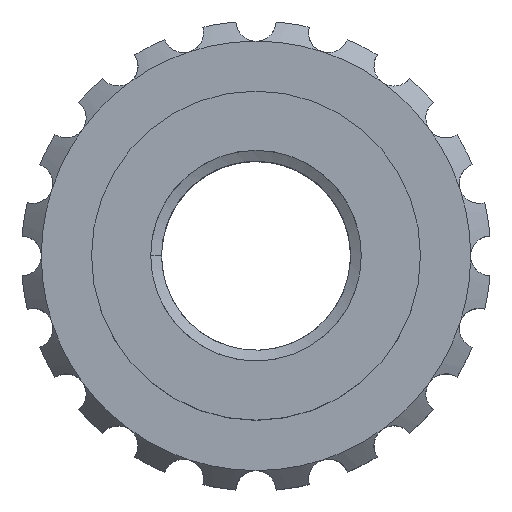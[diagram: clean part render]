
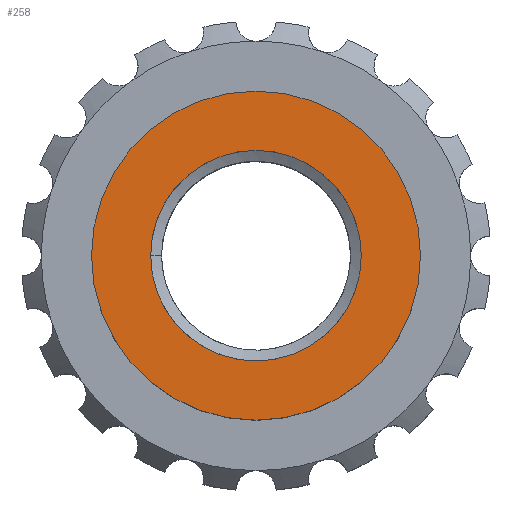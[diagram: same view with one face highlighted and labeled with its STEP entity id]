
A CAD part, top view. The second image highlights one B-rep face of the part: STEP entity #258.
In plain terms, the highlighted planar face has unit normal (0, 0, 1).
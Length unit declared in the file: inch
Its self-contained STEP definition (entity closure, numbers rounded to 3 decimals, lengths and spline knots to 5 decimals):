
#20 = CARTESIAN_POINT ( 'NONE',  ( -1.7725, 0.56133, 0.35 ) ) ;
#68 = CIRCLE ( 'NONE', #2266, 0.13125 ) ;
#102 = EDGE_LOOP ( 'NONE', ( #2602, #1004 ) ) ;
#134 = CIRCLE ( 'NONE', #5142, 0.205 ) ;
#252 = AXIS2_PLACEMENT_3D ( 'NONE', #20, #4884, #3136 ) ;
#258 = ADVANCED_FACE ( 'NONE', ( #4101, #1609 ), #3184, .T. ) ;
#305 = CIRCLE ( 'NONE', #1596, 0.13125 ) ;
#438 = DIRECTION ( 'NONE',  ( 1., 0., 0. ) ) ;
#486 = EDGE_CURVE ( 'NONE', #5292, #3871, #134, .T. ) ;
#491 = DIRECTION ( 'NONE',  ( 1., 0., 0. ) ) ;
#549 = DIRECTION ( 'NONE',  ( 0., 0., 1. ) ) ;
#670 = EDGE_CURVE ( 'NONE', #4198, #3482, #68, .T. ) ;
#1004 = ORIENTED_EDGE ( 'NONE', *, *, #2639, .T. ) ;
#1024 = DIRECTION ( 'NONE',  ( 0., 0., 1. ) ) ;
#1103 = DIRECTION ( 'NONE',  ( 1., 0., 0. ) ) ;
#1596 = AXIS2_PLACEMENT_3D ( 'NONE', #4904, #3501, #438 ) ;
#1609 = FACE_BOUND ( 'NONE', #2058, .T. ) ;
#2058 = EDGE_LOOP ( 'NONE', ( #3765, #2797 ) ) ;
#2060 = DIRECTION ( 'NONE',  ( 1., 0., 0. ) ) ;
#2266 = AXIS2_PLACEMENT_3D ( 'NONE', #4985, #549, #491 ) ;
#2602 = ORIENTED_EDGE ( 'NONE', *, *, #486, .T. ) ;
#2639 = EDGE_CURVE ( 'NONE', #3871, #5292, #3699, .T. ) ;
#2747 = CARTESIAN_POINT ( 'NONE',  ( -1.5675, 0.56133, 0.35 ) ) ;
#2797 = ORIENTED_EDGE ( 'NONE', *, *, #670, .F. ) ;
#2900 = CARTESIAN_POINT ( 'NONE',  ( -1.90375, 0.56133, 0.35 ) ) ;
#2928 = EDGE_CURVE ( 'NONE', #3482, #4198, #305, .T. ) ;
#3065 = CARTESIAN_POINT ( 'NONE',  ( -1.9775, 0.56133, 0.35 ) ) ;
#3136 = DIRECTION ( 'NONE',  ( 1., 0., 0. ) ) ;
#3184 = PLANE ( 'NONE',  #252 ) ;
#3482 = VERTEX_POINT ( 'NONE', #2900 ) ;
#3501 = DIRECTION ( 'NONE',  ( 0., 0., 1. ) ) ;
#3699 = CIRCLE ( 'NONE', #4480, 0.205 ) ;
#3765 = ORIENTED_EDGE ( 'NONE', *, *, #2928, .F. ) ;
#3784 = CARTESIAN_POINT ( 'NONE',  ( -1.64125, 0.56133, 0.35 ) ) ;
#3871 = VERTEX_POINT ( 'NONE', #2747 ) ;
#4101 = FACE_OUTER_BOUND ( 'NONE', #102, .T. ) ;
#4198 = VERTEX_POINT ( 'NONE', #3784 ) ;
#4239 = CARTESIAN_POINT ( 'NONE',  ( -1.7725, 0.56133, 0.35 ) ) ;
#4480 = AXIS2_PLACEMENT_3D ( 'NONE', #5043, #1024, #1103 ) ;
#4884 = DIRECTION ( 'NONE',  ( 0., 0., 1. ) ) ;
#4904 = CARTESIAN_POINT ( 'NONE',  ( -1.7725, 0.56133, 0.35 ) ) ;
#4985 = CARTESIAN_POINT ( 'NONE',  ( -1.7725, 0.56133, 0.35 ) ) ;
#5043 = CARTESIAN_POINT ( 'NONE',  ( -1.7725, 0.56133, 0.35 ) ) ;
#5136 = DIRECTION ( 'NONE',  ( 0., 0., 1. ) ) ;
#5142 = AXIS2_PLACEMENT_3D ( 'NONE', #4239, #5136, #2060 ) ;
#5292 = VERTEX_POINT ( 'NONE', #3065 ) ;
